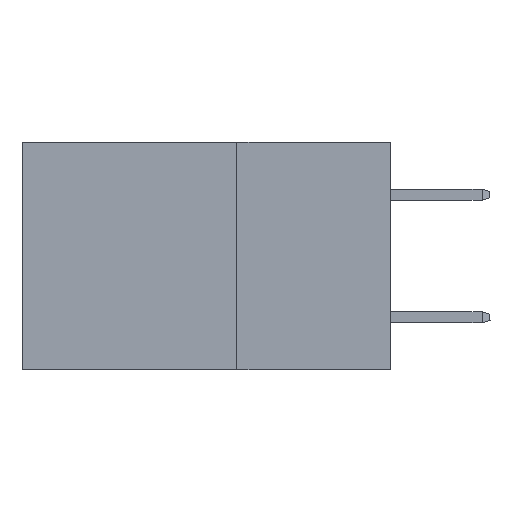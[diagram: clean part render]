
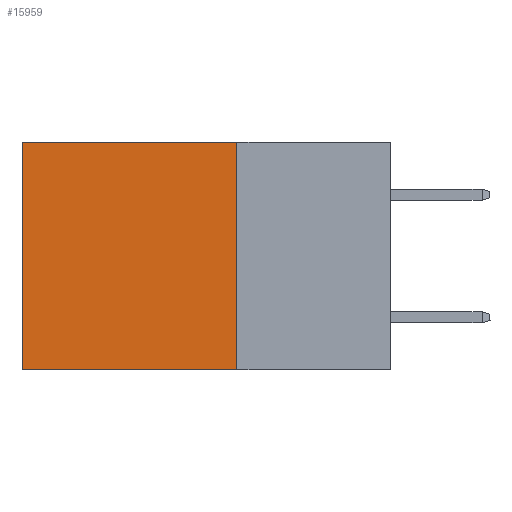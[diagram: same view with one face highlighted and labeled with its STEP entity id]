
A CAD part, left-side view. The second image highlights one B-rep face of the part: STEP entity #15959.
In plain terms, the highlighted planar face has unit normal (-1, 0, 0).
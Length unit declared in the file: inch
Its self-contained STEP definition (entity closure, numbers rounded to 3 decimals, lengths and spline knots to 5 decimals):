
#463 = DIRECTION ( 'NONE',  ( 1., 0., 0. ) ) ;
#4171 = CARTESIAN_POINT ( 'NONE',  ( 0.2875, 0.6, 0. ) ) ;
#4843 = LINE ( 'NONE', #27332, #5772 ) ;
#5157 = CARTESIAN_POINT ( 'NONE',  ( 0.2875, 0.6, -0.37 ) ) ;
#5211 = VERTEX_POINT ( 'NONE', #5157 ) ;
#5772 = VECTOR ( 'NONE', #32897, 39.37008 ) ;
#7253 = CARTESIAN_POINT ( 'NONE',  ( 0.2875, 0.25, 0. ) ) ;
#7617 = ORIENTED_EDGE ( 'NONE', *, *, #34026, .F. ) ;
#12646 = LINE ( 'NONE', #7253, #16705 ) ;
#13123 = EDGE_LOOP ( 'NONE', ( #35408, #7617, #26956, #23824 ) ) ;
#13401 = VERTEX_POINT ( 'NONE', #14873 ) ;
#13736 = EDGE_CURVE ( 'NONE', #13401, #23390, #15935, .T. ) ;
#14709 = VECTOR ( 'NONE', #23756, 39.37008 ) ;
#14803 = VERTEX_POINT ( 'NONE', #4171 ) ;
#14873 = CARTESIAN_POINT ( 'NONE',  ( 0.2875, 0.25, 0. ) ) ;
#15935 = LINE ( 'NONE', #26358, #30502 ) ;
#15959 = ADVANCED_FACE ( 'NONE', ( #27693 ), #32759, .F. ) ;
#16705 = VECTOR ( 'NONE', #22225, 39.37008 ) ;
#17861 = DIRECTION ( 'NONE',  ( 0., 0., -1. ) ) ;
#18843 = CARTESIAN_POINT ( 'NONE',  ( 0.2875, 0.25, -0.37 ) ) ;
#22225 = DIRECTION ( 'NONE',  ( 0., 1., 0. ) ) ;
#23390 = VERTEX_POINT ( 'NONE', #18843 ) ;
#23392 = LINE ( 'NONE', #29454, #14709 ) ;
#23623 = AXIS2_PLACEMENT_3D ( 'NONE', #35662, #463, #27320 ) ;
#23756 = DIRECTION ( 'NONE',  ( 0., 0., -1. ) ) ;
#23824 = ORIENTED_EDGE ( 'NONE', *, *, #30004, .T. ) ;
#25441 = EDGE_CURVE ( 'NONE', #14803, #5211, #23392, .T. ) ;
#26358 = CARTESIAN_POINT ( 'NONE',  ( 0.2875, 0.25, 0. ) ) ;
#26956 = ORIENTED_EDGE ( 'NONE', *, *, #13736, .F. ) ;
#27320 = DIRECTION ( 'NONE',  ( 0., 0., -1. ) ) ;
#27332 = CARTESIAN_POINT ( 'NONE',  ( 0.2875, 0.25, -0.37 ) ) ;
#27693 = FACE_OUTER_BOUND ( 'NONE', #13123, .T. ) ;
#29454 = CARTESIAN_POINT ( 'NONE',  ( 0.2875, 0.6, 0. ) ) ;
#30004 = EDGE_CURVE ( 'NONE', #13401, #14803, #12646, .T. ) ;
#30502 = VECTOR ( 'NONE', #17861, 39.37008 ) ;
#32759 = PLANE ( 'NONE',  #23623 ) ;
#32897 = DIRECTION ( 'NONE',  ( 0., 1., 0. ) ) ;
#34026 = EDGE_CURVE ( 'NONE', #23390, #5211, #4843, .T. ) ;
#35408 = ORIENTED_EDGE ( 'NONE', *, *, #25441, .T. ) ;
#35662 = CARTESIAN_POINT ( 'NONE',  ( 0.2875, 0.25, 0. ) ) ;
